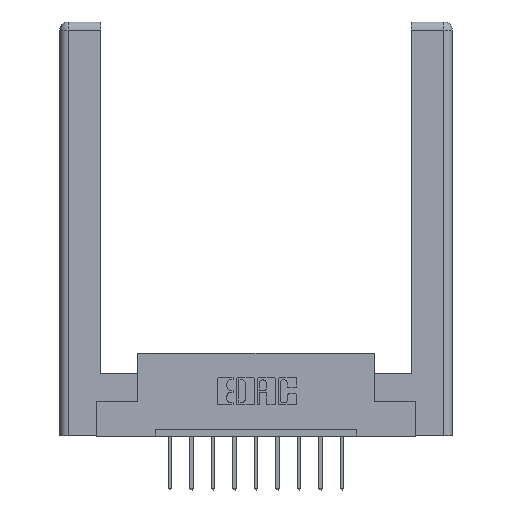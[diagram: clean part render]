
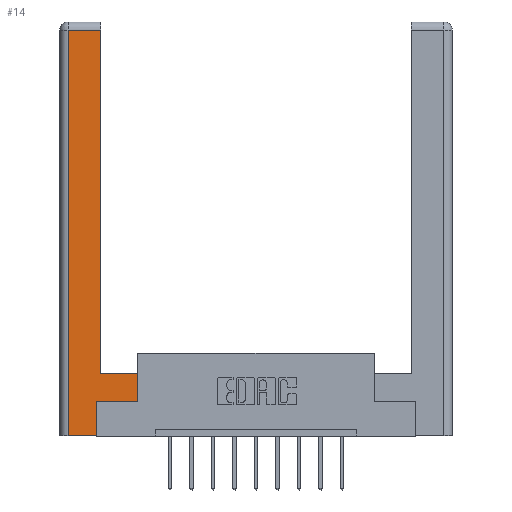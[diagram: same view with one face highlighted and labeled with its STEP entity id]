
A CAD part, top view. The second image highlights one B-rep face of the part: STEP entity #14.
In plain terms, the highlighted planar face has unit normal (0, 0, 1).
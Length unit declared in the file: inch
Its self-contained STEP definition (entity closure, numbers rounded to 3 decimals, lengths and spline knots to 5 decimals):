
#14 = ADVANCED_FACE ( 'NONE', ( #30 ), #3930, .F. ) ;
#30 = FACE_OUTER_BOUND ( 'NONE', #11174, .T. ) ;
#687 = LINE ( 'NONE', #5661, #4170 ) ;
#698 = CARTESIAN_POINT ( 'NONE',  ( 0.265, 0., 0. ) ) ;
#810 = VECTOR ( 'NONE', #10195, 39.37008 ) ;
#1018 = CARTESIAN_POINT ( 'NONE',  ( 0.265, 0.245, 0. ) ) ;
#1109 = ORIENTED_EDGE ( 'NONE', *, *, #2269, .T. ) ;
#1120 = LINE ( 'NONE', #9573, #9640 ) ;
#1399 = EDGE_CURVE ( 'NONE', #10043, #6509, #11660, .T. ) ;
#1486 = LINE ( 'NONE', #698, #810 ) ;
#1591 = DIRECTION ( 'NONE',  ( -1., 0., 0. ) ) ;
#2042 = DIRECTION ( 'NONE',  ( -1., 0., 0. ) ) ;
#2269 = EDGE_CURVE ( 'NONE', #5496, #10043, #1120, .T. ) ;
#2582 = DIRECTION ( 'NONE',  ( 0., 1., 0. ) ) ;
#3110 = VERTEX_POINT ( 'NONE', #10676 ) ;
#3129 = VECTOR ( 'NONE', #10298, 39.37008 ) ;
#3387 = VERTEX_POINT ( 'NONE', #5254 ) ;
#3544 = DIRECTION ( 'NONE',  ( -1., 0., 0. ) ) ;
#3619 = CARTESIAN_POINT ( 'NONE',  ( 0.0615, 2.94, 0. ) ) ;
#3930 = PLANE ( 'NONE',  #13482 ) ;
#3932 = ORIENTED_EDGE ( 'NONE', *, *, #5074, .T. ) ;
#4008 = LINE ( 'NONE', #13162, #8441 ) ;
#4170 = VECTOR ( 'NONE', #3544, 39.37008 ) ;
#4759 = ORIENTED_EDGE ( 'NONE', *, *, #10148, .T. ) ;
#5074 = EDGE_CURVE ( 'NONE', #3110, #11627, #1486, .T. ) ;
#5254 = CARTESIAN_POINT ( 'NONE',  ( 0.295, 2.94, 0. ) ) ;
#5496 = VERTEX_POINT ( 'NONE', #7244 ) ;
#5661 = CARTESIAN_POINT ( 'NONE',  ( 0.0615, 2.94, 0. ) ) ;
#6228 = DIRECTION ( 'NONE',  ( 0., 0., -1. ) ) ;
#6334 = CARTESIAN_POINT ( 'NONE',  ( 0.565, 0.245, 0. ) ) ;
#6425 = ORIENTED_EDGE ( 'NONE', *, *, #6495, .T. ) ;
#6456 = VECTOR ( 'NONE', #9474, 39.37008 ) ;
#6495 = EDGE_CURVE ( 'NONE', #6509, #3387, #9796, .T. ) ;
#6509 = VERTEX_POINT ( 'NONE', #12353 ) ;
#7011 = DIRECTION ( 'NONE',  ( 0., -1., 0. ) ) ;
#7016 = CARTESIAN_POINT ( 'NONE',  ( 0.265, 0.245, 0. ) ) ;
#7237 = LINE ( 'NONE', #7016, #3129 ) ;
#7244 = CARTESIAN_POINT ( 'NONE',  ( 0.565, 0.245, 0. ) ) ;
#7305 = DIRECTION ( 'NONE',  ( 0., 1., 0. ) ) ;
#8441 = VECTOR ( 'NONE', #7011, 39.37008 ) ;
#8592 = ORIENTED_EDGE ( 'NONE', *, *, #11656, .T. ) ;
#8714 = ORIENTED_EDGE ( 'NONE', *, *, #12854, .T. ) ;
#8856 = VECTOR ( 'NONE', #1591, 39.37008 ) ;
#9474 = DIRECTION ( 'NONE',  ( 1., 0., 0. ) ) ;
#9573 = CARTESIAN_POINT ( 'NONE',  ( 0.565, 0.45, 0. ) ) ;
#9640 = VECTOR ( 'NONE', #7305, 39.37008 ) ;
#9796 = LINE ( 'NONE', #13158, #13444 ) ;
#10043 = VERTEX_POINT ( 'NONE', #13233 ) ;
#10148 = EDGE_CURVE ( 'NONE', #11270, #3110, #4008, .T. ) ;
#10195 = DIRECTION ( 'NONE',  ( 1., 0., 0. ) ) ;
#10209 = LINE ( 'NONE', #6334, #6456 ) ;
#10298 = DIRECTION ( 'NONE',  ( 0., 1., 0. ) ) ;
#10676 = CARTESIAN_POINT ( 'NONE',  ( 0.0615, 0., 0. ) ) ;
#11165 = CARTESIAN_POINT ( 'NONE',  ( 0.295, 0.45, 0. ) ) ;
#11174 = EDGE_LOOP ( 'NONE', ( #6425, #8592, #4759, #3932, #8714, #13582, #1109, #12061 ) ) ;
#11267 = CARTESIAN_POINT ( 'NONE',  ( 0., 0., 0. ) ) ;
#11270 = VERTEX_POINT ( 'NONE', #3619 ) ;
#11552 = CARTESIAN_POINT ( 'NONE',  ( 0.265, 0., 0. ) ) ;
#11627 = VERTEX_POINT ( 'NONE', #11552 ) ;
#11656 = EDGE_CURVE ( 'NONE', #3387, #11270, #687, .T. ) ;
#11660 = LINE ( 'NONE', #11165, #8856 ) ;
#11906 = EDGE_CURVE ( 'NONE', #13085, #5496, #10209, .T. ) ;
#12061 = ORIENTED_EDGE ( 'NONE', *, *, #1399, .T. ) ;
#12353 = CARTESIAN_POINT ( 'NONE',  ( 0.295, 0.45, 0. ) ) ;
#12854 = EDGE_CURVE ( 'NONE', #11627, #13085, #7237, .T. ) ;
#13085 = VERTEX_POINT ( 'NONE', #1018 ) ;
#13158 = CARTESIAN_POINT ( 'NONE',  ( 0.295, 3., 0. ) ) ;
#13162 = CARTESIAN_POINT ( 'NONE',  ( 0.0615, 0., 0. ) ) ;
#13233 = CARTESIAN_POINT ( 'NONE',  ( 0.565, 0.45, 0. ) ) ;
#13444 = VECTOR ( 'NONE', #2582, 39.37008 ) ;
#13482 = AXIS2_PLACEMENT_3D ( 'NONE', #11267, #6228, #2042 ) ;
#13582 = ORIENTED_EDGE ( 'NONE', *, *, #11906, .T. ) ;
